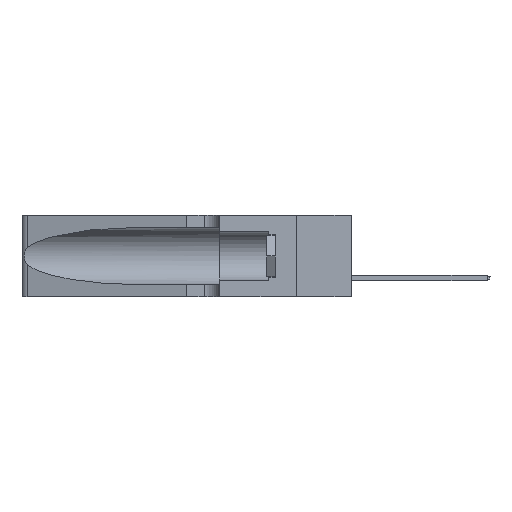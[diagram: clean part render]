
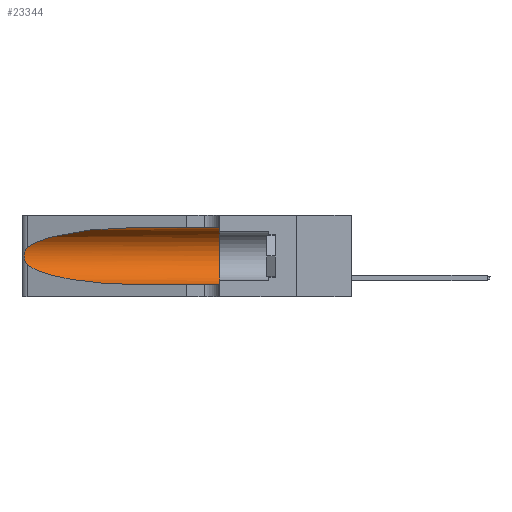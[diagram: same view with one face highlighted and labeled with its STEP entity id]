
A CAD part, left-side view. The second image highlights one B-rep face of the part: STEP entity #23344.
In plain terms, the highlighted cylindrical face has radius 3.308 mm (diameter 6.617 mm), a partial arc.
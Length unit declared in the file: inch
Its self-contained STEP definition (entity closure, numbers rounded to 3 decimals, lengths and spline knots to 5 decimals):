
#239 = VERTEX_POINT ( 'NONE', #27252 ) ;
#334 = ORIENTED_EDGE ( 'NONE', *, *, #21630, .F. ) ;
#900 = CARTESIAN_POINT ( 'NONE',  ( 0.18966, 0.96281, 0.05475 ) ) ;
#1268 = CARTESIAN_POINT ( 'NONE',  ( 0.1305, 0.72297, 0.05475 ) ) ;
#1473 = CARTESIAN_POINT ( 'NONE',  ( 0.1305, 1.61858, 0.185 ) ) ;
#3463 = ORIENTED_EDGE ( 'NONE', *, *, #13392, .T. ) ;
#3603 = B_SPLINE_CURVE_WITH_KNOTS ( 'NONE', 3,
 ( #14336, #46969, #42840, #43151, #23482, #35509, #50414, #23331, #31434, #28132, #12346, #43301, #5193, #32054 ),
 .UNSPECIFIED., .F., .F.,
 ( 4, 2, 2, 2, 2, 2, 4 ),
 ( 0., 0.00027, 0.00053, 0.00107, 0.0016, 0.00187, 0.00214 ),
 .UNSPECIFIED. ) ;
#5193 = CARTESIAN_POINT ( 'NONE',  ( 0.25555, 1.22993, 0.14849 ) ) ;
#7473 = CARTESIAN_POINT ( 'NONE',  ( 0.1305, 0.72297, 0.05475 ) ) ;
#10958 = EDGE_CURVE ( 'NONE', #16972, #43241, #16285, .T. ) ;
#12064 = CIRCLE ( 'NONE', #25058, 0.13025 ) ;
#12067 = VECTOR ( 'NONE', #14135, 39.37008 ) ;
#12346 = CARTESIAN_POINT ( 'NONE',  ( 0.25789, 1.23486, 0.15765 ) ) ;
#13216 = CARTESIAN_POINT ( 'NONE',  ( 0.1305, 0.35, 0.31525 ) ) ;
#13392 = EDGE_CURVE ( 'NONE', #28229, #239, #25279, .T. ) ;
#14135 = DIRECTION ( 'NONE',  ( 0., -1., 0. ) ) ;
#14178 =( BOUNDED_CURVE ( )  B_SPLINE_CURVE ( 3, ( #14705, #44571, #900, #1268 ),
 .UNSPECIFIED., .F., .F. ) 
 B_SPLINE_CURVE_WITH_KNOTS ( ( 4, 4 ),
 ( 3.44316, 4.71239 ),
 .UNSPECIFIED. ) 
 CURVE ( )  GEOMETRIC_REPRESENTATION_ITEM ( )  RATIONAL_B_SPLINE_CURVE ( ( 1., 0.87, 0.87, 1. ) ) 
 REPRESENTATION_ITEM ( '' )  );
#14336 = CARTESIAN_POINT ( 'NONE',  ( 0.25487, 1.22718, 0.22369 ) ) ;
#14705 = CARTESIAN_POINT ( 'NONE',  ( 0.25487, 1.22718, 0.14631 ) ) ;
#15480 = CARTESIAN_POINT ( 'NONE',  ( 0.25487, 1.22718, 0.14631 ) ) ;
#16285 = LINE ( 'NONE', #43662, #12067 ) ;
#16972 = VERTEX_POINT ( 'NONE', #33941 ) ;
#18991 = AXIS2_PLACEMENT_3D ( 'NONE', #1473, #21473, #28747 ) ;
#21473 = DIRECTION ( 'NONE',  ( 0., -1., 0. ) ) ;
#21630 = EDGE_CURVE ( 'NONE', #43241, #239, #12064, .T. ) ;
#23331 = CARTESIAN_POINT ( 'NONE',  ( 0.26075, 1.23896, 0.178 ) ) ;
#23344 = ADVANCED_FACE ( 'NONE', ( #36215 ), #35087, .F. ) ;
#23482 = CARTESIAN_POINT ( 'NONE',  ( 0.25854, 1.2359, 0.20912 ) ) ;
#23613 = CARTESIAN_POINT ( 'NONE',  ( 0.25487, 1.22718, 0.22369 ) ) ;
#25058 = AXIS2_PLACEMENT_3D ( 'NONE', #48456, #28851, #40949 ) ;
#25279 = LINE ( 'NONE', #32206, #27688 ) ;
#27252 = CARTESIAN_POINT ( 'NONE',  ( 0.1305, 0.35, 0.05475 ) ) ;
#27688 = VECTOR ( 'NONE', #36837, 39.37008 ) ;
#28132 = CARTESIAN_POINT ( 'NONE',  ( 0.25856, 1.23593, 0.16098 ) ) ;
#28229 = VERTEX_POINT ( 'NONE', #7473 ) ;
#28747 = DIRECTION ( 'NONE',  ( 0., 0., -1. ) ) ;
#28851 = DIRECTION ( 'NONE',  ( 0., 1., 0. ) ) ;
#29552 = CARTESIAN_POINT ( 'NONE',  ( 0.2373, 1.15595, 0.28018 ) ) ;
#30313 = ORIENTED_EDGE ( 'NONE', *, *, #10958, .F. ) ;
#31434 = CARTESIAN_POINT ( 'NONE',  ( 0.26017, 1.23833, 0.17102 ) ) ;
#32054 = CARTESIAN_POINT ( 'NONE',  ( 0.25487, 1.22718, 0.14631 ) ) ;
#32206 = CARTESIAN_POINT ( 'NONE',  ( 0.1305, 1.61858, 0.05475 ) ) ;
#32959 = EDGE_CURVE ( 'NONE', #16972, #48811, #37530, .T. ) ;
#33333 = CARTESIAN_POINT ( 'NONE',  ( 0.25487, 1.22718, 0.22369 ) ) ;
#33941 = CARTESIAN_POINT ( 'NONE',  ( 0.1305, 0.72297, 0.31525 ) ) ;
#34707 = EDGE_CURVE ( 'NONE', #47329, #28229, #14178, .T. ) ;
#35087 = CYLINDRICAL_SURFACE ( 'NONE', #18991, 0.13025 ) ;
#35509 = CARTESIAN_POINT ( 'NONE',  ( 0.26018, 1.23835, 0.19895 ) ) ;
#36215 = FACE_OUTER_BOUND ( 'NONE', #45462, .T. ) ;
#36837 = DIRECTION ( 'NONE',  ( 0., -1., 0. ) ) ;
#36881 = ORIENTED_EDGE ( 'NONE', *, *, #34707, .T. ) ;
#37530 =( BOUNDED_CURVE ( )  B_SPLINE_CURVE ( 3, ( #50277, #40549, #29552, #33333 ),
 .UNSPECIFIED., .F., .F. ) 
 B_SPLINE_CURVE_WITH_KNOTS ( ( 4, 4 ),
 ( 1.5708, 2.84003 ),
 .UNSPECIFIED. ) 
 CURVE ( )  GEOMETRIC_REPRESENTATION_ITEM ( )  RATIONAL_B_SPLINE_CURVE ( ( 1., 0.87, 0.87, 1. ) ) 
 REPRESENTATION_ITEM ( '' )  );
#38389 = ORIENTED_EDGE ( 'NONE', *, *, #43242, .T. ) ;
#40474 = ORIENTED_EDGE ( 'NONE', *, *, #32959, .T. ) ;
#40549 = CARTESIAN_POINT ( 'NONE',  ( 0.18966, 0.96281, 0.31525 ) ) ;
#40949 = DIRECTION ( 'NONE',  ( 0., 0., 1. ) ) ;
#42840 = CARTESIAN_POINT ( 'NONE',  ( 0.25639, 1.23184, 0.21858 ) ) ;
#43151 = CARTESIAN_POINT ( 'NONE',  ( 0.25787, 1.23484, 0.2124 ) ) ;
#43241 = VERTEX_POINT ( 'NONE', #13216 ) ;
#43242 = EDGE_CURVE ( 'NONE', #48811, #47329, #3603, .T. ) ;
#43301 = CARTESIAN_POINT ( 'NONE',  ( 0.25639, 1.23186, 0.15144 ) ) ;
#43662 = CARTESIAN_POINT ( 'NONE',  ( 0.1305, 1.61858, 0.31525 ) ) ;
#44571 = CARTESIAN_POINT ( 'NONE',  ( 0.2373, 1.15595, 0.08982 ) ) ;
#45462 = EDGE_LOOP ( 'NONE', ( #40474, #38389, #36881, #3463, #334, #30313 ) ) ;
#46969 = CARTESIAN_POINT ( 'NONE',  ( 0.25555, 1.22994, 0.2215 ) ) ;
#47329 = VERTEX_POINT ( 'NONE', #15480 ) ;
#48456 = CARTESIAN_POINT ( 'NONE',  ( 0.1305, 0.35, 0.185 ) ) ;
#48811 = VERTEX_POINT ( 'NONE', #23613 ) ;
#50277 = CARTESIAN_POINT ( 'NONE',  ( 0.1305, 0.72297, 0.31525 ) ) ;
#50414 = CARTESIAN_POINT ( 'NONE',  ( 0.26075, 1.23896, 0.19203 ) ) ;
